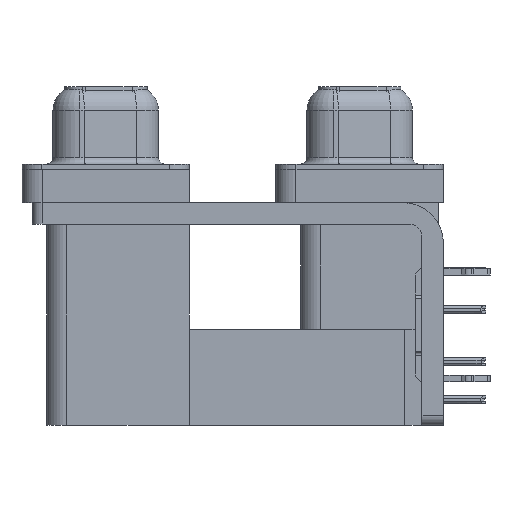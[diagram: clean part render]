
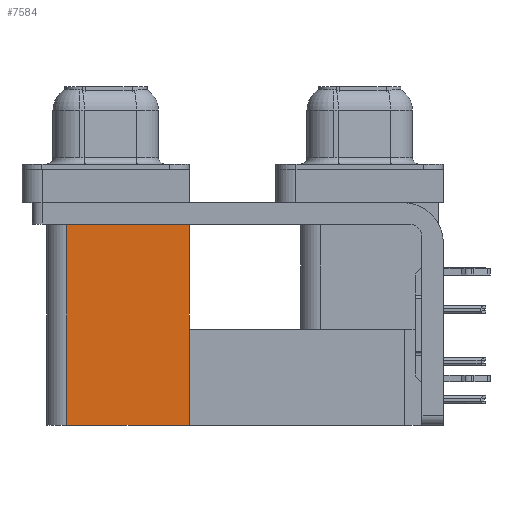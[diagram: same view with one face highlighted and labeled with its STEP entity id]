
A CAD part, left-side view. The second image highlights one B-rep face of the part: STEP entity #7584.
In plain terms, the highlighted planar face has unit normal (-1, 0, 0).
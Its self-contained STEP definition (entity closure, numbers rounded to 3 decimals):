
#79 = DIRECTION ( 'NONE',  ( 0., 1., 0. ) ) ;
#586 = DIRECTION ( 'NONE',  ( 0., 0., -1. ) ) ;
#1769 = EDGE_CURVE ( 'NONE', #48674, #6624, #48183, .T. ) ;
#2134 = EDGE_LOOP ( 'NONE', ( #4733, #47265, #31232, #5562 ) ) ;
#4216 = LINE ( 'NONE', #27903, #18492 ) ;
#4295 = EDGE_CURVE ( 'NONE', #11730, #6624, #21166, .T. ) ;
#4566 = VECTOR ( 'NONE', #79, 1000. ) ;
#4733 = ORIENTED_EDGE ( 'NONE', *, *, #4295, .T. ) ;
#5562 = ORIENTED_EDGE ( 'NONE', *, *, #44743, .T. ) ;
#6624 = VERTEX_POINT ( 'NONE', #19228 ) ;
#7584 = ADVANCED_FACE ( 'NONE', ( #15715 ), #47741, .F. ) ;
#11730 = VERTEX_POINT ( 'NONE', #40792 ) ;
#11973 = VERTEX_POINT ( 'NONE', #25962 ) ;
#15715 = FACE_OUTER_BOUND ( 'NONE', #2134, .T. ) ;
#16044 = AXIS2_PLACEMENT_3D ( 'NONE', #36488, #36245, #586 ) ;
#17200 = VECTOR ( 'NONE', #32551, 1000. ) ;
#18492 = VECTOR ( 'NONE', #46960, 1000. ) ;
#18572 = EDGE_CURVE ( 'NONE', #11973, #48674, #34711, .T. ) ;
#19228 = CARTESIAN_POINT ( 'NONE',  ( 3.765, 21.975, -2.5 ) ) ;
#21166 = LINE ( 'NONE', #40160, #4566 ) ;
#25962 = CARTESIAN_POINT ( 'NONE',  ( 3.765, 12.775, -19.2 ) ) ;
#27903 = CARTESIAN_POINT ( 'NONE',  ( 3.765, 12.775, -19.2 ) ) ;
#31232 = ORIENTED_EDGE ( 'NONE', *, *, #18572, .F. ) ;
#32551 = DIRECTION ( 'NONE',  ( 0., 0., 1. ) ) ;
#34711 = LINE ( 'NONE', #42769, #36709 ) ;
#36245 = DIRECTION ( 'NONE',  ( 1., 0., 0. ) ) ;
#36488 = CARTESIAN_POINT ( 'NONE',  ( 3.765, 12.775, -19.2 ) ) ;
#36709 = VECTOR ( 'NONE', #38858, 1000. ) ;
#38858 = DIRECTION ( 'NONE',  ( 0., 1., 0. ) ) ;
#40160 = CARTESIAN_POINT ( 'NONE',  ( 3.765, 12.775, -2.5 ) ) ;
#40792 = CARTESIAN_POINT ( 'NONE',  ( 3.765, 12.775, -2.5 ) ) ;
#42165 = CARTESIAN_POINT ( 'NONE',  ( 3.765, 21.975, -19.2 ) ) ;
#42769 = CARTESIAN_POINT ( 'NONE',  ( 3.765, 12.775, -19.2 ) ) ;
#44743 = EDGE_CURVE ( 'NONE', #11973, #11730, #4216, .T. ) ;
#46960 = DIRECTION ( 'NONE',  ( 0., 0., 1. ) ) ;
#47265 = ORIENTED_EDGE ( 'NONE', *, *, #1769, .F. ) ;
#47741 = PLANE ( 'NONE',  #16044 ) ;
#48183 = LINE ( 'NONE', #48450, #17200 ) ;
#48450 = CARTESIAN_POINT ( 'NONE',  ( 3.765, 21.975, -19.2 ) ) ;
#48674 = VERTEX_POINT ( 'NONE', #42165 ) ;
